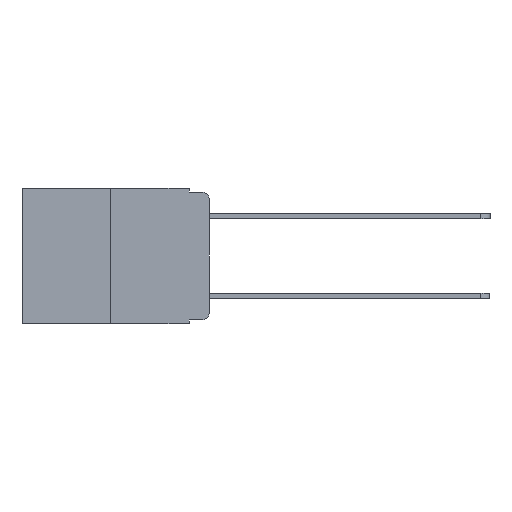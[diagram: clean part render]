
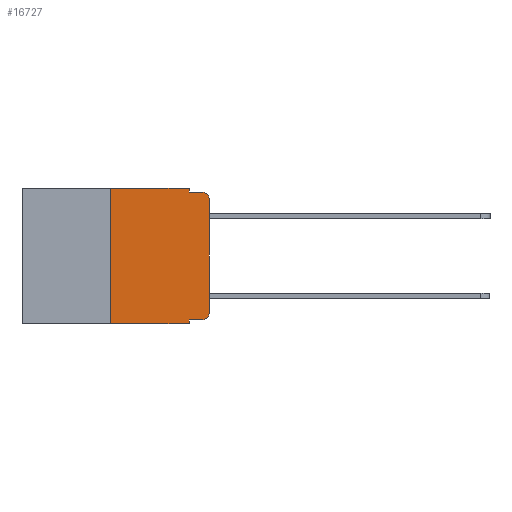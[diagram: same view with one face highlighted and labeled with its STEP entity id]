
A CAD part, left-side view. The second image highlights one B-rep face of the part: STEP entity #16727.
In plain terms, the highlighted planar face has unit normal (-1, 0, 0).
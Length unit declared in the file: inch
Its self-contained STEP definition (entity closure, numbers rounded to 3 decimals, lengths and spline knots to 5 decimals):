
#456 = ORIENTED_EDGE ( 'NONE', *, *, #18391, .F. ) ;
#595 = CARTESIAN_POINT ( 'NONE',  ( 0., 0.473, 0. ) ) ;
#622 = ORIENTED_EDGE ( 'NONE', *, *, #5328, .T. ) ;
#717 = ORIENTED_EDGE ( 'NONE', *, *, #17194, .T. ) ;
#1013 = CARTESIAN_POINT ( 'NONE',  ( 0., 0., -0.03 ) ) ;
#1209 = LINE ( 'NONE', #6313, #8658 ) ;
#1237 = ORIENTED_EDGE ( 'NONE', *, *, #7625, .F. ) ;
#1252 = CARTESIAN_POINT ( 'NONE',  ( 0., 0.051, -0.01 ) ) ;
#1534 = EDGE_CURVE ( 'NONE', #9750, #17688, #13550, .T. ) ;
#1635 = VERTEX_POINT ( 'NONE', #1997 ) ;
#1690 = ORIENTED_EDGE ( 'NONE', *, *, #5003, .T. ) ;
#1912 = VECTOR ( 'NONE', #15475, 39.37008 ) ;
#1997 = CARTESIAN_POINT ( 'NONE',  ( 0., 0.051, 0. ) ) ;
#2190 = EDGE_CURVE ( 'NONE', #18164, #17688, #14175, .T. ) ;
#2195 = ORIENTED_EDGE ( 'NONE', *, *, #1534, .F. ) ;
#2390 = EDGE_CURVE ( 'NONE', #6891, #4177, #11204, .T. ) ;
#2900 = LINE ( 'NONE', #13192, #10145 ) ;
#2907 = DIRECTION ( 'NONE',  ( 0., 0., 1. ) ) ;
#3082 = DIRECTION ( 'NONE',  ( 0., -1., 0. ) ) ;
#3348 = VECTOR ( 'NONE', #3082, 39.37008 ) ;
#3626 = DIRECTION ( 'NONE',  ( 0., 0., -1. ) ) ;
#4177 = VERTEX_POINT ( 'NONE', #1013 ) ;
#4516 = DIRECTION ( 'NONE',  ( -1., 0., 0. ) ) ;
#5003 = EDGE_CURVE ( 'NONE', #10656, #6891, #6063, .T. ) ;
#5181 = ORIENTED_EDGE ( 'NONE', *, *, #2190, .T. ) ;
#5328 = EDGE_CURVE ( 'NONE', #4177, #5517, #11891, .T. ) ;
#5406 = ORIENTED_EDGE ( 'NONE', *, *, #16512, .F. ) ;
#5481 = VERTEX_POINT ( 'NONE', #16494 ) ;
#5517 = VERTEX_POINT ( 'NONE', #13831 ) ;
#5830 = DIRECTION ( 'NONE',  ( 0., 0., -1. ) ) ;
#6063 = CIRCLE ( 'NONE', #15482, 0.02 ) ;
#6072 = ORIENTED_EDGE ( 'NONE', *, *, #16977, .F. ) ;
#6313 = CARTESIAN_POINT ( 'NONE',  ( 0., 0.051, -0.333 ) ) ;
#6367 = ORIENTED_EDGE ( 'NONE', *, *, #2390, .T. ) ;
#6471 = CARTESIAN_POINT ( 'NONE',  ( 0., 0.25, 0. ) ) ;
#6573 = DIRECTION ( 'NONE',  ( -1., 0., 0. ) ) ;
#6638 = FACE_OUTER_BOUND ( 'NONE', #11016, .T. ) ;
#6749 = DIRECTION ( 'NONE',  ( 1., 0., 0. ) ) ;
#6853 = VECTOR ( 'NONE', #18232, 39.37008 ) ;
#6891 = VERTEX_POINT ( 'NONE', #18292 ) ;
#7231 = CARTESIAN_POINT ( 'NONE',  ( 0., 0.02, -0.313 ) ) ;
#7513 = VECTOR ( 'NONE', #2907, 39.37008 ) ;
#7625 = EDGE_CURVE ( 'NONE', #16169, #1635, #14162, .T. ) ;
#7668 = CARTESIAN_POINT ( 'NONE',  ( 0., 0., 0. ) ) ;
#8649 = CARTESIAN_POINT ( 'NONE',  ( 0., 0.051, 0. ) ) ;
#8658 = VECTOR ( 'NONE', #11872, 39.37008 ) ;
#8878 = VECTOR ( 'NONE', #5830, 39.37008 ) ;
#9750 = VERTEX_POINT ( 'NONE', #11969 ) ;
#10002 = CARTESIAN_POINT ( 'NONE',  ( 0., 0.25, -0.343 ) ) ;
#10145 = VECTOR ( 'NONE', #14581, 39.37008 ) ;
#10210 = DIRECTION ( 'NONE',  ( 0., 0., -1. ) ) ;
#10656 = VERTEX_POINT ( 'NONE', #13899 ) ;
#11016 = EDGE_LOOP ( 'NONE', ( #6367, #622, #5406, #6072, #1237, #456, #5181, #2195, #717, #1690 ) ) ;
#11204 = LINE ( 'NONE', #7668, #7513 ) ;
#11646 = CARTESIAN_POINT ( 'NONE',  ( 0., 0.473, 0. ) ) ;
#11872 = DIRECTION ( 'NONE',  ( 0., -1., 0. ) ) ;
#11891 = CIRCLE ( 'NONE', #16976, 0.02 ) ;
#11969 = CARTESIAN_POINT ( 'NONE',  ( 0., 0.051, -0.333 ) ) ;
#12246 = PLANE ( 'NONE',  #17234 ) ;
#12515 = LINE ( 'NONE', #8649, #8878 ) ;
#13192 = CARTESIAN_POINT ( 'NONE',  ( 0., 0.25, 0. ) ) ;
#13310 = LINE ( 'NONE', #1252, #1912 ) ;
#13550 = LINE ( 'NONE', #16354, #17206 ) ;
#13831 = CARTESIAN_POINT ( 'NONE',  ( 0., 0.02, -0.01 ) ) ;
#13899 = CARTESIAN_POINT ( 'NONE',  ( 0., 0.02, -0.333 ) ) ;
#14162 = LINE ( 'NONE', #11646, #3348 ) ;
#14175 = LINE ( 'NONE', #18230, #6853 ) ;
#14581 = DIRECTION ( 'NONE',  ( 0., 0., 1. ) ) ;
#14819 = CARTESIAN_POINT ( 'NONE',  ( 0., 0.02, -0.03 ) ) ;
#15475 = DIRECTION ( 'NONE',  ( 0., -1., 0. ) ) ;
#15482 = AXIS2_PLACEMENT_3D ( 'NONE', #7231, #4516, #10210 ) ;
#16169 = VERTEX_POINT ( 'NONE', #6471 ) ;
#16198 = DIRECTION ( 'NONE',  ( 0., 0., -1. ) ) ;
#16354 = CARTESIAN_POINT ( 'NONE',  ( 0., 0.051, 0. ) ) ;
#16369 = DIRECTION ( 'NONE',  ( 0., 0., -1. ) ) ;
#16494 = CARTESIAN_POINT ( 'NONE',  ( 0., 0.051, -0.01 ) ) ;
#16512 = EDGE_CURVE ( 'NONE', #5481, #5517, #13310, .T. ) ;
#16727 = ADVANCED_FACE ( 'NONE', ( #6638 ), #12246, .F. ) ;
#16976 = AXIS2_PLACEMENT_3D ( 'NONE', #14819, #6573, #16198 ) ;
#16977 = EDGE_CURVE ( 'NONE', #1635, #5481, #12515, .T. ) ;
#17194 = EDGE_CURVE ( 'NONE', #9750, #10656, #1209, .T. ) ;
#17206 = VECTOR ( 'NONE', #3626, 39.37008 ) ;
#17234 = AXIS2_PLACEMENT_3D ( 'NONE', #595, #6749, #16369 ) ;
#17688 = VERTEX_POINT ( 'NONE', #18487 ) ;
#18164 = VERTEX_POINT ( 'NONE', #10002 ) ;
#18230 = CARTESIAN_POINT ( 'NONE',  ( 0., 0.473, -0.343 ) ) ;
#18232 = DIRECTION ( 'NONE',  ( 0., -1., 0. ) ) ;
#18292 = CARTESIAN_POINT ( 'NONE',  ( 0., 0., -0.313 ) ) ;
#18391 = EDGE_CURVE ( 'NONE', #18164, #16169, #2900, .T. ) ;
#18487 = CARTESIAN_POINT ( 'NONE',  ( 0., 0.051, -0.343 ) ) ;
